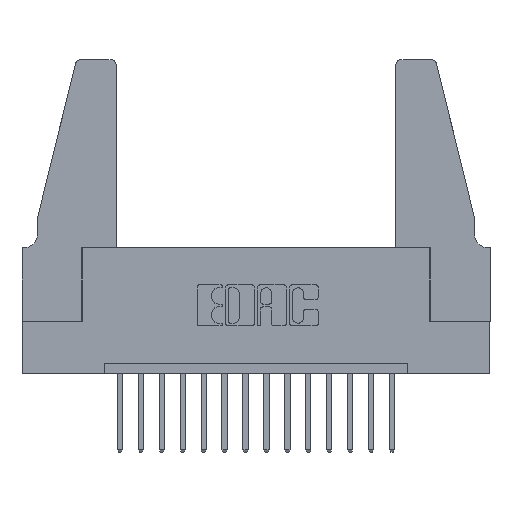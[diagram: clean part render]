
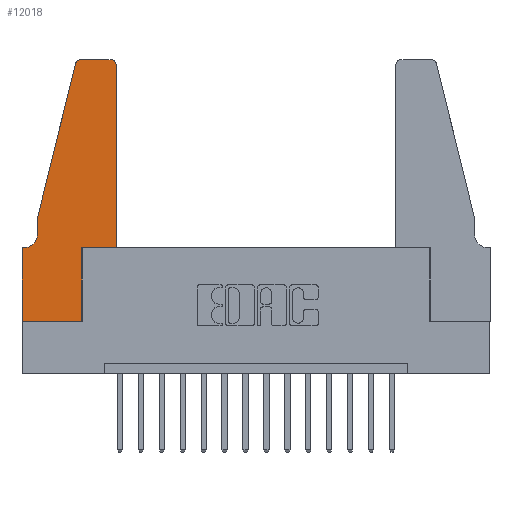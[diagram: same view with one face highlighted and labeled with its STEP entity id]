
A CAD part, top view. The second image highlights one B-rep face of the part: STEP entity #12018.
In plain terms, the highlighted planar face has unit normal (0, 0, 1).
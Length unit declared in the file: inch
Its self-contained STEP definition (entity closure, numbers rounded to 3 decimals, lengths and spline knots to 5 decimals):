
#56 = EDGE_CURVE ( 'NONE', #9512, #14603, #4581, .T. ) ;
#476 = ORIENTED_EDGE ( 'NONE', *, *, #10053, .T. ) ;
#698 = CARTESIAN_POINT ( 'NONE',  ( 0.2865, 0., 0.37 ) ) ;
#709 = AXIS2_PLACEMENT_3D ( 'NONE', #13792, #10064, #4936 ) ;
#738 = VECTOR ( 'NONE', #2352, 39.37008 ) ;
#801 = CARTESIAN_POINT ( 'NONE',  ( 0.4505, 0.35, 0.37 ) ) ;
#991 = CARTESIAN_POINT ( 'NONE',  ( 0.0755, 0.35, 0.37 ) ) ;
#1109 = CARTESIAN_POINT ( 'NONE',  ( 0.25487, 1.22718, 0.37 ) ) ;
#1356 = DIRECTION ( 'NONE',  ( 0., -1., 0. ) ) ;
#1446 = VECTOR ( 'NONE', #14841, 39.37008 ) ;
#1487 = LINE ( 'NONE', #16356, #14622 ) ;
#1540 = ORIENTED_EDGE ( 'NONE', *, *, #3059, .T. ) ;
#1586 = VERTEX_POINT ( 'NONE', #1109 ) ;
#1593 = EDGE_CURVE ( 'NONE', #1586, #8732, #1487, .T. ) ;
#1766 = DIRECTION ( 'NONE',  ( 0., 0., -1. ) ) ;
#1810 = EDGE_CURVE ( 'NONE', #15754, #1586, #5528, .T. ) ;
#1902 = CARTESIAN_POINT ( 'NONE',  ( 0.284, 1.22, 0.37 ) ) ;
#2352 = DIRECTION ( 'NONE',  ( 1., 0., 0. ) ) ;
#2422 = DIRECTION ( 'NONE',  ( -1., 0., 0. ) ) ;
#2692 = VERTEX_POINT ( 'NONE', #5432 ) ;
#2723 = VECTOR ( 'NONE', #1356, 39.37008 ) ;
#2743 = LINE ( 'NONE', #6203, #15456 ) ;
#2744 = EDGE_CURVE ( 'NONE', #6477, #10578, #8080, .T. ) ;
#2749 = CARTESIAN_POINT ( 'NONE',  ( 0.0755, 0.42, 0.37 ) ) ;
#2784 = DIRECTION ( 'NONE',  ( 1., 0., 0. ) ) ;
#2868 = VECTOR ( 'NONE', #13700, 39.37008 ) ;
#2967 = LINE ( 'NONE', #6136, #738 ) ;
#3059 = EDGE_CURVE ( 'NONE', #10537, #15754, #16148, .T. ) ;
#3088 = CARTESIAN_POINT ( 'NONE',  ( 0.0755, 0.5, 0.37 ) ) ;
#3845 = EDGE_CURVE ( 'NONE', #5708, #6477, #2743, .T. ) ;
#3979 = CARTESIAN_POINT ( 'NONE',  ( 0., 0., 0.37 ) ) ;
#4161 = AXIS2_PLACEMENT_3D ( 'NONE', #1902, #5746, #15796 ) ;
#4251 = DIRECTION ( 'NONE',  ( -1., 0., 0. ) ) ;
#4318 = CARTESIAN_POINT ( 'NONE',  ( 0.0055, 0.42, 0.37 ) ) ;
#4352 = CARTESIAN_POINT ( 'NONE',  ( 0.0755, 0.5, 0.37 ) ) ;
#4581 = CIRCLE ( 'NONE', #11562, 0.07 ) ;
#4936 = DIRECTION ( 'NONE',  ( 1., 0., 0. ) ) ;
#5336 = EDGE_CURVE ( 'NONE', #10578, #6644, #11704, .T. ) ;
#5432 = CARTESIAN_POINT ( 'NONE',  ( 0., 0., 0.37 ) ) ;
#5528 = CIRCLE ( 'NONE', #4161, 0.03 ) ;
#5574 = DIRECTION ( 'NONE',  ( 0., -1., 0. ) ) ;
#5617 = CARTESIAN_POINT ( 'NONE',  ( 0., 0.35, 0.37 ) ) ;
#5708 = VERTEX_POINT ( 'NONE', #698 ) ;
#5746 = DIRECTION ( 'NONE',  ( 0., 0., 1. ) ) ;
#5809 = ORIENTED_EDGE ( 'NONE', *, *, #6020, .T. ) ;
#6020 = EDGE_CURVE ( 'NONE', #8732, #9512, #8907, .T. ) ;
#6136 = CARTESIAN_POINT ( 'NONE',  ( 0., 0., 0.37 ) ) ;
#6203 = CARTESIAN_POINT ( 'NONE',  ( 0.2865, 0.35, 0.37 ) ) ;
#6339 = CARTESIAN_POINT ( 'NONE',  ( 0.2865, 0.35, 0.37 ) ) ;
#6349 = EDGE_LOOP ( 'NONE', ( #1540, #15314, #14955, #5809, #15788, #7291, #476, #12657, #7319, #7220, #10205, #15147 ) ) ;
#6477 = VERTEX_POINT ( 'NONE', #6339 ) ;
#6644 = VERTEX_POINT ( 'NONE', #11078 ) ;
#6892 = EDGE_CURVE ( 'NONE', #14603, #9529, #13806, .T. ) ;
#7220 = ORIENTED_EDGE ( 'NONE', *, *, #2744, .T. ) ;
#7291 = ORIENTED_EDGE ( 'NONE', *, *, #6892, .T. ) ;
#7319 = ORIENTED_EDGE ( 'NONE', *, *, #3845, .T. ) ;
#7472 = VECTOR ( 'NONE', #2422, 39.37008 ) ;
#7668 = DIRECTION ( 'NONE',  ( 0., 1., 0. ) ) ;
#7681 = AXIS2_PLACEMENT_3D ( 'NONE', #10347, #12862, #2784 ) ;
#7685 = CARTESIAN_POINT ( 'NONE',  ( 0.0055, 0.35, 0.37 ) ) ;
#8080 = LINE ( 'NONE', #801, #1446 ) ;
#8515 = VECTOR ( 'NONE', #5574, 39.37008 ) ;
#8732 = VERTEX_POINT ( 'NONE', #3088 ) ;
#8800 = DIRECTION ( 'NONE',  ( -0.239, -0.971, 0. ) ) ;
#8907 = LINE ( 'NONE', #4352, #8515 ) ;
#9001 = EDGE_CURVE ( 'NONE', #6644, #10537, #9972, .T. ) ;
#9413 = FACE_OUTER_BOUND ( 'NONE', #6349, .T. ) ;
#9508 = VECTOR ( 'NONE', #7668, 39.37008 ) ;
#9512 = VERTEX_POINT ( 'NONE', #2749 ) ;
#9529 = VERTEX_POINT ( 'NONE', #5617 ) ;
#9962 = PLANE ( 'NONE',  #709 ) ;
#9972 = CIRCLE ( 'NONE', #7681, 0.03 ) ;
#10053 = EDGE_CURVE ( 'NONE', #9529, #2692, #12481, .T. ) ;
#10064 = DIRECTION ( 'NONE',  ( 0., 0., 1. ) ) ;
#10205 = ORIENTED_EDGE ( 'NONE', *, *, #5336, .T. ) ;
#10347 = CARTESIAN_POINT ( 'NONE',  ( 0.4205, 1.22, 0.37 ) ) ;
#10537 = VERTEX_POINT ( 'NONE', #14528 ) ;
#10578 = VERTEX_POINT ( 'NONE', #12728 ) ;
#11078 = CARTESIAN_POINT ( 'NONE',  ( 0.4505, 1.22, 0.37 ) ) ;
#11562 = AXIS2_PLACEMENT_3D ( 'NONE', #4318, #1766, #4251 ) ;
#11704 = LINE ( 'NONE', #15241, #9508 ) ;
#12018 = ADVANCED_FACE ( 'NONE', ( #9413 ), #9962, .T. ) ;
#12481 = LINE ( 'NONE', #3979, #2723 ) ;
#12616 = DIRECTION ( 'NONE',  ( 0., 1., 0. ) ) ;
#12657 = ORIENTED_EDGE ( 'NONE', *, *, #14484, .T. ) ;
#12728 = CARTESIAN_POINT ( 'NONE',  ( 0.4505, 0.35, 0.37 ) ) ;
#12862 = DIRECTION ( 'NONE',  ( 0., 0., 1. ) ) ;
#13700 = DIRECTION ( 'NONE',  ( -1., 0., 0. ) ) ;
#13792 = CARTESIAN_POINT ( 'NONE',  ( 0., 0.35, 0.37 ) ) ;
#13806 = LINE ( 'NONE', #991, #2868 ) ;
#14484 = EDGE_CURVE ( 'NONE', #2692, #5708, #2967, .T. ) ;
#14528 = CARTESIAN_POINT ( 'NONE',  ( 0.4205, 1.25, 0.37 ) ) ;
#14603 = VERTEX_POINT ( 'NONE', #7685 ) ;
#14622 = VECTOR ( 'NONE', #8800, 39.37008 ) ;
#14739 = CARTESIAN_POINT ( 'NONE',  ( 0.284, 1.25, 0.37 ) ) ;
#14841 = DIRECTION ( 'NONE',  ( 1., 0., 0. ) ) ;
#14955 = ORIENTED_EDGE ( 'NONE', *, *, #1593, .T. ) ;
#15049 = CARTESIAN_POINT ( 'NONE',  ( 0.2605, 1.25, 0.37 ) ) ;
#15147 = ORIENTED_EDGE ( 'NONE', *, *, #9001, .T. ) ;
#15241 = CARTESIAN_POINT ( 'NONE',  ( 0.4505, 0.35, 0.37 ) ) ;
#15314 = ORIENTED_EDGE ( 'NONE', *, *, #1810, .T. ) ;
#15456 = VECTOR ( 'NONE', #12616, 39.37008 ) ;
#15754 = VERTEX_POINT ( 'NONE', #14739 ) ;
#15788 = ORIENTED_EDGE ( 'NONE', *, *, #56, .T. ) ;
#15796 = DIRECTION ( 'NONE',  ( 1., 0., 0. ) ) ;
#16148 = LINE ( 'NONE', #15049, #7472 ) ;
#16356 = CARTESIAN_POINT ( 'NONE',  ( 0.0755, 0.5, 0.37 ) ) ;
